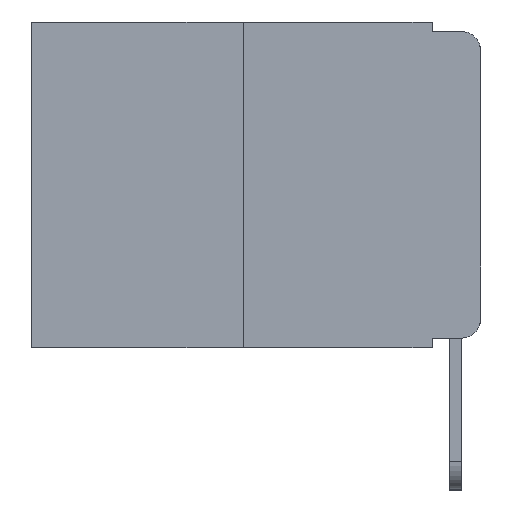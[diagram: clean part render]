
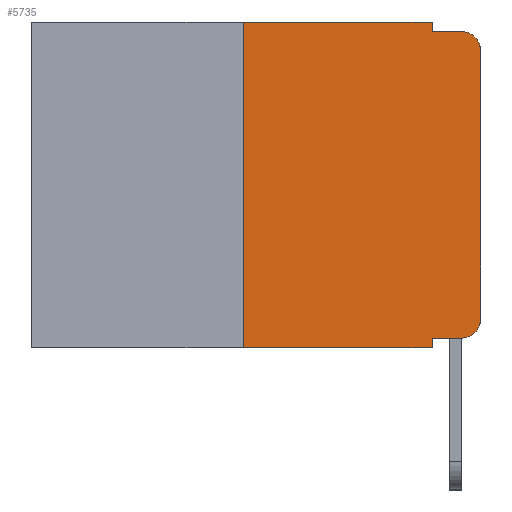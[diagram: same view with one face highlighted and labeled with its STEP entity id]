
A CAD part, left-side view. The second image highlights one B-rep face of the part: STEP entity #5735.
In plain terms, the highlighted planar face has unit normal (-1, 0, 0).
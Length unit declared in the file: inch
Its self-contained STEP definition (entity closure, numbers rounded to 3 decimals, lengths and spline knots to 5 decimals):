
#15 = CARTESIAN_POINT ( 'NONE',  ( 0., 0., -0.03 ) ) ;
#52 = DIRECTION ( 'NONE',  ( -1., 0., 0. ) ) ;
#80 = CARTESIAN_POINT ( 'NONE',  ( 0., 0.02, -0.313 ) ) ;
#155 = VERTEX_POINT ( 'NONE', #1923 ) ;
#293 = CARTESIAN_POINT ( 'NONE',  ( 0., 0.051, -0.333 ) ) ;
#818 = ORIENTED_EDGE ( 'NONE', *, *, #2938, .F. ) ;
#835 = CARTESIAN_POINT ( 'NONE',  ( 0., 0.473, -0.343 ) ) ;
#917 = DIRECTION ( 'NONE',  ( -1., 0., 0. ) ) ;
#1146 = LINE ( 'NONE', #293, #6046 ) ;
#1212 = ORIENTED_EDGE ( 'NONE', *, *, #7893, .F. ) ;
#1430 = CARTESIAN_POINT ( 'NONE',  ( 0., 0., -0.313 ) ) ;
#1573 = ORIENTED_EDGE ( 'NONE', *, *, #2111, .F. ) ;
#1621 = LINE ( 'NONE', #10256, #8663 ) ;
#1701 = CARTESIAN_POINT ( 'NONE',  ( 0., 0.051, -0.343 ) ) ;
#1923 = CARTESIAN_POINT ( 'NONE',  ( 0., 0.25, 0. ) ) ;
#1968 = VERTEX_POINT ( 'NONE', #10915 ) ;
#2018 = DIRECTION ( 'NONE',  ( 0., 0., -1. ) ) ;
#2025 = VERTEX_POINT ( 'NONE', #2883 ) ;
#2111 = EDGE_CURVE ( 'NONE', #11676, #4482, #3941, .T. ) ;
#2406 = CARTESIAN_POINT ( 'NONE',  ( 0., 0.25, -0.343 ) ) ;
#2503 = CARTESIAN_POINT ( 'NONE',  ( 0., 0.051, -0.01 ) ) ;
#2568 = DIRECTION ( 'NONE',  ( 0., 0., -1. ) ) ;
#2615 = EDGE_CURVE ( 'NONE', #2025, #6703, #6413, .T. ) ;
#2721 = VECTOR ( 'NONE', #9761, 39.37008 ) ;
#2787 = VERTEX_POINT ( 'NONE', #15 ) ;
#2883 = CARTESIAN_POINT ( 'NONE',  ( 0., 0.051, 0. ) ) ;
#2933 = EDGE_CURVE ( 'NONE', #5338, #155, #11456, .T. ) ;
#2938 = EDGE_CURVE ( 'NONE', #6703, #1968, #1621, .T. ) ;
#2951 = EDGE_CURVE ( 'NONE', #2787, #1968, #6401, .T. ) ;
#3111 = DIRECTION ( 'NONE',  ( 0., 0., -1. ) ) ;
#3331 = ORIENTED_EDGE ( 'NONE', *, *, #3565, .T. ) ;
#3365 = DIRECTION ( 'NONE',  ( 0., -1., 0. ) ) ;
#3565 = EDGE_CURVE ( 'NONE', #10924, #2787, #5294, .T. ) ;
#3651 = ORIENTED_EDGE ( 'NONE', *, *, #2615, .F. ) ;
#3681 = CARTESIAN_POINT ( 'NONE',  ( 0., 0., 0. ) ) ;
#3941 = LINE ( 'NONE', #3987, #8359 ) ;
#3965 = CARTESIAN_POINT ( 'NONE',  ( 0., 0.051, 0. ) ) ;
#3987 = CARTESIAN_POINT ( 'NONE',  ( 0., 0.051, 0. ) ) ;
#4482 = VERTEX_POINT ( 'NONE', #1701 ) ;
#4784 = CIRCLE ( 'NONE', #6263, 0.02 ) ;
#4943 = DIRECTION ( 'NONE',  ( 0., -1., 0. ) ) ;
#5176 = DIRECTION ( 'NONE',  ( 0., 0., 1. ) ) ;
#5234 = CARTESIAN_POINT ( 'NONE',  ( 0., 0.02, -0.03 ) ) ;
#5294 = LINE ( 'NONE', #3681, #2721 ) ;
#5338 = VERTEX_POINT ( 'NONE', #2406 ) ;
#5700 = DIRECTION ( 'NONE',  ( 0., -1., 0. ) ) ;
#5728 = AXIS2_PLACEMENT_3D ( 'NONE', #8831, #8931, #9111 ) ;
#5735 = ADVANCED_FACE ( 'NONE', ( #7964 ), #9012, .F. ) ;
#6046 = VECTOR ( 'NONE', #3365, 39.37008 ) ;
#6092 = DIRECTION ( 'NONE',  ( 0., -1., 0. ) ) ;
#6263 = AXIS2_PLACEMENT_3D ( 'NONE', #80, #52, #3111 ) ;
#6356 = ORIENTED_EDGE ( 'NONE', *, *, #2933, .F. ) ;
#6401 = CIRCLE ( 'NONE', #8942, 0.02 ) ;
#6413 = LINE ( 'NONE', #3965, #8677 ) ;
#6703 = VERTEX_POINT ( 'NONE', #2503 ) ;
#6886 = ORIENTED_EDGE ( 'NONE', *, *, #8209, .T. ) ;
#6915 = VECTOR ( 'NONE', #4943, 39.37008 ) ;
#7524 = VECTOR ( 'NONE', #6092, 39.37008 ) ;
#7600 = CARTESIAN_POINT ( 'NONE',  ( 0., 0.25, 0. ) ) ;
#7893 = EDGE_CURVE ( 'NONE', #155, #2025, #12020, .T. ) ;
#7964 = FACE_OUTER_BOUND ( 'NONE', #9434, .T. ) ;
#7969 = VERTEX_POINT ( 'NONE', #8631 ) ;
#8102 = ORIENTED_EDGE ( 'NONE', *, *, #2951, .T. ) ;
#8209 = EDGE_CURVE ( 'NONE', #7969, #10924, #4784, .T. ) ;
#8257 = EDGE_CURVE ( 'NONE', #11676, #7969, #1146, .T. ) ;
#8359 = VECTOR ( 'NONE', #2568, 39.37008 ) ;
#8631 = CARTESIAN_POINT ( 'NONE',  ( 0., 0.02, -0.333 ) ) ;
#8663 = VECTOR ( 'NONE', #5700, 39.37008 ) ;
#8677 = VECTOR ( 'NONE', #2018, 39.37008 ) ;
#8831 = CARTESIAN_POINT ( 'NONE',  ( 0., 0.473, 0. ) ) ;
#8931 = DIRECTION ( 'NONE',  ( 1., 0., 0. ) ) ;
#8939 = VECTOR ( 'NONE', #5176, 39.37008 ) ;
#8942 = AXIS2_PLACEMENT_3D ( 'NONE', #5234, #917, #9423 ) ;
#9012 = PLANE ( 'NONE',  #5728 ) ;
#9111 = DIRECTION ( 'NONE',  ( 0., 0., -1. ) ) ;
#9196 = LINE ( 'NONE', #835, #6915 ) ;
#9423 = DIRECTION ( 'NONE',  ( 0., 0., -1. ) ) ;
#9434 = EDGE_LOOP ( 'NONE', ( #3331, #8102, #818, #3651, #1212, #6356, #10868, #1573, #11133, #6886 ) ) ;
#9699 = CARTESIAN_POINT ( 'NONE',  ( 0., 0.473, 0. ) ) ;
#9761 = DIRECTION ( 'NONE',  ( 0., 0., 1. ) ) ;
#9978 = CARTESIAN_POINT ( 'NONE',  ( 0., 0.051, -0.333 ) ) ;
#10256 = CARTESIAN_POINT ( 'NONE',  ( 0., 0.051, -0.01 ) ) ;
#10868 = ORIENTED_EDGE ( 'NONE', *, *, #11130, .T. ) ;
#10915 = CARTESIAN_POINT ( 'NONE',  ( 0., 0.02, -0.01 ) ) ;
#10924 = VERTEX_POINT ( 'NONE', #1430 ) ;
#11130 = EDGE_CURVE ( 'NONE', #5338, #4482, #9196, .T. ) ;
#11133 = ORIENTED_EDGE ( 'NONE', *, *, #8257, .T. ) ;
#11456 = LINE ( 'NONE', #7600, #8939 ) ;
#11676 = VERTEX_POINT ( 'NONE', #9978 ) ;
#12020 = LINE ( 'NONE', #9699, #7524 ) ;
